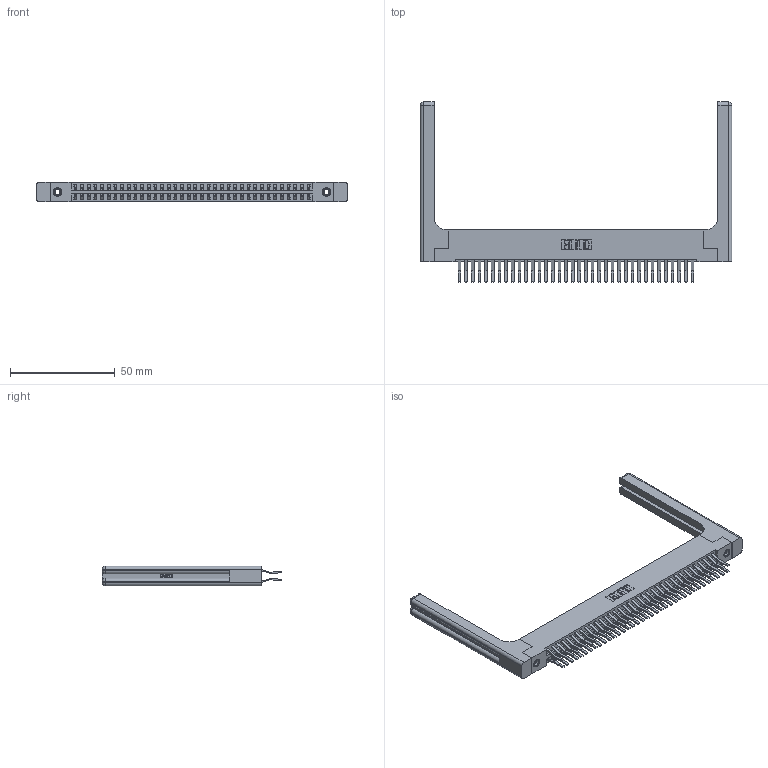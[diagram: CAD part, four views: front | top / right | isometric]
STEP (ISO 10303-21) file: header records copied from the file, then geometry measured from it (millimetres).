
FILE_DESCRIPTION (( 'STEP AP203' ), '1' );
FILE_NAME ('396-072-560-258.STEP', '2019-10-30T20:24:46', ( '' ), ( '' ), 'SwSTEP 2.0', 'SolidWorks 2016', '' );
FILE_SCHEMA (( 'CONFIG_CONTROL_DESIGN' ));
Length unit declared in the file: inch
Products named in the file (5): 345-292-001_560 Tail; 345-250-001_345-250-001-102; 346-220-058_345-220-058; 346 Part_Flush Mounting Lugs - 0.156 Dia-TH; 396-072-560-258
Assembly tree (77 placements, depth 2):
  396-072-560-258
    346 Part_Flush Mounting Lugs - 0.156 Dia-TH
    345-292-001_560 Tail  x72
    345-250-001_345-250-001-102  x2
    346-220-058_345-220-058  x2
Bounding box: 148.36 x 85.74 x 9.4 mm (x, y, z)
Volume: 22386.7 mm3; surface area: 26608.2 mm2
Topology: 77 solids, 77 shells, 4266 faces, 12587 edges, 8274 vertices
Faces by surface type: plane 2744, cylinder 1462, bspline 36, cone 12, sphere 8, torus 4
Entity records: 29572 total; most frequent: CARTESIAN_POINT 5889, ORIENTED_EDGE 4620, DIRECTION 4178, EDGE_CURVE 2310, VECTOR 1938, LINE 1938, VERTEX_POINT 1530, AXIS2_PLACEMENT_3D 1120
